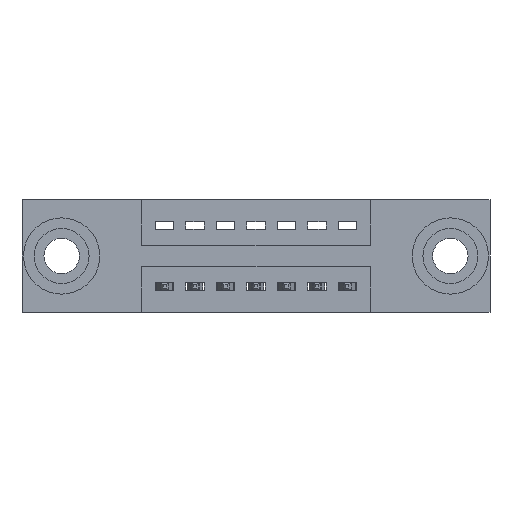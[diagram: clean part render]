
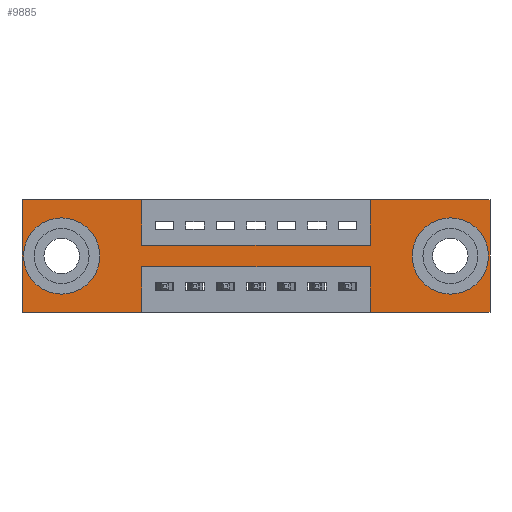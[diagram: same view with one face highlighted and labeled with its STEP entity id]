
A CAD part, front view. The second image highlights one B-rep face of the part: STEP entity #9885.
In plain terms, the highlighted planar face has unit normal (0, -1, 0).
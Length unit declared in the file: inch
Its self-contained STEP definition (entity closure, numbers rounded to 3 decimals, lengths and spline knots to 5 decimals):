
#82 = VERTEX_POINT ( 'NONE', #1654 ) ;
#415 = EDGE_CURVE ( 'NONE', #9062, #1113, #5996, .T. ) ;
#456 = ORIENTED_EDGE ( 'NONE', *, *, #10142, .F. ) ;
#490 = CARTESIAN_POINT ( 'NONE',  ( 0.13, 0., -0.263 ) ) ;
#629 = VERTEX_POINT ( 'NONE', #3877 ) ;
#755 = DIRECTION ( 'NONE',  ( 0., 0., -1. ) ) ;
#882 = VECTOR ( 'NONE', #6548, 39.37008 ) ;
#938 = CARTESIAN_POINT ( 'NONE',  ( 0.3925, 0., -0.15 ) ) ;
#989 = VERTEX_POINT ( 'NONE', #1128 ) ;
#1016 = DIRECTION ( 'NONE',  ( 0., 0., -1. ) ) ;
#1083 = ORIENTED_EDGE ( 'NONE', *, *, #5784, .F. ) ;
#1094 = CARTESIAN_POINT ( 'NONE',  ( 1.1425, 0., -0.22 ) ) ;
#1100 = AXIS2_PLACEMENT_3D ( 'NONE', #1557, #7455, #2564 ) ;
#1113 = VERTEX_POINT ( 'NONE', #490 ) ;
#1128 = CARTESIAN_POINT ( 'NONE',  ( 1.405, 0., -0.107 ) ) ;
#1370 = CARTESIAN_POINT ( 'NONE',  ( 1.1425, 0., -0.37 ) ) ;
#1557 = CARTESIAN_POINT ( 'NONE',  ( 1.405, 0., -0.185 ) ) ;
#1654 = CARTESIAN_POINT ( 'NONE',  ( 0.3925, 0., -0.22 ) ) ;
#1697 = VECTOR ( 'NONE', #1016, 39.37008 ) ;
#1730 = VERTEX_POINT ( 'NONE', #938 ) ;
#1739 = EDGE_CURVE ( 'NONE', #4841, #6452, #4478, .T. ) ;
#1789 = VECTOR ( 'NONE', #4950, 39.37008 ) ;
#1843 = CIRCLE ( 'NONE', #1100, 0.078 ) ;
#2000 = VECTOR ( 'NONE', #4420, 39.37008 ) ;
#2006 = FACE_BOUND ( 'NONE', #2363, .T. ) ;
#2059 = EDGE_LOOP ( 'NONE', ( #9842, #8125, #456, #5400, #7371, #9270, #5641, #1083, #9943, #5024, #2950, #7493 ) ) ;
#2079 = DIRECTION ( 'NONE',  ( 0., 1., 0. ) ) ;
#2245 = CARTESIAN_POINT ( 'NONE',  ( 0., 0., 0. ) ) ;
#2363 = EDGE_LOOP ( 'NONE', ( #2468, #4809 ) ) ;
#2468 = ORIENTED_EDGE ( 'NONE', *, *, #7388, .T. ) ;
#2542 = CARTESIAN_POINT ( 'NONE',  ( 0., 0., -0.37 ) ) ;
#2557 = VERTEX_POINT ( 'NONE', #5149 ) ;
#2564 = DIRECTION ( 'NONE',  ( 0., 0., -1. ) ) ;
#2681 = EDGE_CURVE ( 'NONE', #82, #2557, #8882, .T. ) ;
#2788 = CARTESIAN_POINT ( 'NONE',  ( 1.1425, 0., 0. ) ) ;
#2950 = ORIENTED_EDGE ( 'NONE', *, *, #9751, .F. ) ;
#2962 = DIRECTION ( 'NONE',  ( 0., 1., 0. ) ) ;
#3237 = EDGE_CURVE ( 'NONE', #2557, #629, #6519, .T. ) ;
#3473 = AXIS2_PLACEMENT_3D ( 'NONE', #7750, #2962, #8460 ) ;
#3496 = AXIS2_PLACEMENT_3D ( 'NONE', #6977, #9857, #5509 ) ;
#3508 = CARTESIAN_POINT ( 'NONE',  ( 1.535, 0., 0. ) ) ;
#3595 = CARTESIAN_POINT ( 'NONE',  ( 0., 0., 0. ) ) ;
#3743 = DIRECTION ( 'NONE',  ( 0., 0., 1. ) ) ;
#3753 = CARTESIAN_POINT ( 'NONE',  ( 1.535, 0., 0. ) ) ;
#3757 = DIRECTION ( 'NONE',  ( 0., 1., 0. ) ) ;
#3770 = CARTESIAN_POINT ( 'NONE',  ( 0.13, 0., -0.185 ) ) ;
#3877 = CARTESIAN_POINT ( 'NONE',  ( 0., 0., -0.37 ) ) ;
#3926 = AXIS2_PLACEMENT_3D ( 'NONE', #3770, #3757, #3743 ) ;
#4138 = VERTEX_POINT ( 'NONE', #1094 ) ;
#4142 = CARTESIAN_POINT ( 'NONE',  ( 0.3925, 0., -0.22 ) ) ;
#4152 = CARTESIAN_POINT ( 'NONE',  ( 0.3925, 0., -0.37 ) ) ;
#4199 = FACE_BOUND ( 'NONE', #8728, .T. ) ;
#4329 = EDGE_CURVE ( 'NONE', #6452, #5755, #8646, .T. ) ;
#4360 = CARTESIAN_POINT ( 'NONE',  ( 1.1425, 0., 0. ) ) ;
#4420 = DIRECTION ( 'NONE',  ( -1., 0., 0. ) ) ;
#4478 = LINE ( 'NONE', #3508, #1697 ) ;
#4557 = LINE ( 'NONE', #5351, #1789 ) ;
#4621 = VECTOR ( 'NONE', #9121, 39.37008 ) ;
#4710 = PLANE ( 'NONE',  #3496 ) ;
#4809 = ORIENTED_EDGE ( 'NONE', *, *, #9693, .T. ) ;
#4841 = VERTEX_POINT ( 'NONE', #3753 ) ;
#4912 = VECTOR ( 'NONE', #9776, 39.37008 ) ;
#4950 = DIRECTION ( 'NONE',  ( 1., 0., 0. ) ) ;
#4968 = DIRECTION ( 'NONE',  ( -1., 0., 0. ) ) ;
#5024 = ORIENTED_EDGE ( 'NONE', *, *, #8645, .F. ) ;
#5037 = VERTEX_POINT ( 'NONE', #10582 ) ;
#5149 = CARTESIAN_POINT ( 'NONE',  ( 0.3925, 0., -0.37 ) ) ;
#5194 = DIRECTION ( 'NONE',  ( -1., 0., 0. ) ) ;
#5217 = ORIENTED_EDGE ( 'NONE', *, *, #8427, .T. ) ;
#5263 = LINE ( 'NONE', #3595, #6782 ) ;
#5277 = CARTESIAN_POINT ( 'NONE',  ( 0., 0., 0. ) ) ;
#5351 = CARTESIAN_POINT ( 'NONE',  ( 0.3925, 0., -0.15 ) ) ;
#5400 = ORIENTED_EDGE ( 'NONE', *, *, #4329, .F. ) ;
#5401 = EDGE_CURVE ( 'NONE', #10257, #4841, #9762, .T. ) ;
#5408 = VERTEX_POINT ( 'NONE', #9918 ) ;
#5509 = DIRECTION ( 'NONE',  ( 0., 0., -1. ) ) ;
#5545 = CARTESIAN_POINT ( 'NONE',  ( 1.1425, 0., -0.37 ) ) ;
#5547 = ORIENTED_EDGE ( 'NONE', *, *, #415, .T. ) ;
#5641 = ORIENTED_EDGE ( 'NONE', *, *, #7259, .F. ) ;
#5755 = VERTEX_POINT ( 'NONE', #5545 ) ;
#5784 = EDGE_CURVE ( 'NONE', #1730, #6793, #4557, .T. ) ;
#5996 = CIRCLE ( 'NONE', #3926, 0.078 ) ;
#6452 = VERTEX_POINT ( 'NONE', #10271 ) ;
#6519 = LINE ( 'NONE', #2542, #2000 ) ;
#6548 = DIRECTION ( 'NONE',  ( 0., 0., 1. ) ) ;
#6607 = VECTOR ( 'NONE', #4968, 39.37008 ) ;
#6782 = VECTOR ( 'NONE', #8199, 39.37008 ) ;
#6793 = VERTEX_POINT ( 'NONE', #7779 ) ;
#6933 = LINE ( 'NONE', #2788, #4912 ) ;
#6977 = CARTESIAN_POINT ( 'NONE',  ( 0., 0., -0.37 ) ) ;
#7086 = CARTESIAN_POINT ( 'NONE',  ( 1.405, 0., -0.185 ) ) ;
#7130 = AXIS2_PLACEMENT_3D ( 'NONE', #7086, #2079, #7795 ) ;
#7238 = CARTESIAN_POINT ( 'NONE',  ( 0.13, 0., -0.107 ) ) ;
#7259 = EDGE_CURVE ( 'NONE', #6793, #10257, #6933, .T. ) ;
#7358 = CIRCLE ( 'NONE', #3473, 0.078 ) ;
#7371 = ORIENTED_EDGE ( 'NONE', *, *, #1739, .F. ) ;
#7388 = EDGE_CURVE ( 'NONE', #989, #5408, #7720, .T. ) ;
#7455 = DIRECTION ( 'NONE',  ( 0., 1., 0. ) ) ;
#7493 = ORIENTED_EDGE ( 'NONE', *, *, #3237, .F. ) ;
#7720 = CIRCLE ( 'NONE', #7130, 0.078 ) ;
#7750 = CARTESIAN_POINT ( 'NONE',  ( 0.13, 0., -0.185 ) ) ;
#7779 = CARTESIAN_POINT ( 'NONE',  ( 1.1425, 0., -0.15 ) ) ;
#7795 = DIRECTION ( 'NONE',  ( 0., 0., -1. ) ) ;
#7845 = VECTOR ( 'NONE', #10093, 39.37008 ) ;
#7870 = LINE ( 'NONE', #5277, #9352 ) ;
#8125 = ORIENTED_EDGE ( 'NONE', *, *, #10658, .F. ) ;
#8181 = VECTOR ( 'NONE', #5194, 39.37008 ) ;
#8199 = DIRECTION ( 'NONE',  ( 1., 0., 0. ) ) ;
#8203 = FACE_OUTER_BOUND ( 'NONE', #2059, .T. ) ;
#8337 = LINE ( 'NONE', #8424, #4621 ) ;
#8424 = CARTESIAN_POINT ( 'NONE',  ( 0.3925, 0., 0. ) ) ;
#8427 = EDGE_CURVE ( 'NONE', #1113, #9062, #7358, .T. ) ;
#8460 = DIRECTION ( 'NONE',  ( 0., 0., 1. ) ) ;
#8522 = LINE ( 'NONE', #4142, #6607 ) ;
#8645 = EDGE_CURVE ( 'NONE', #10647, #5037, #5263, .T. ) ;
#8646 = LINE ( 'NONE', #8901, #8181 ) ;
#8672 = VECTOR ( 'NONE', #755, 39.37008 ) ;
#8728 = EDGE_LOOP ( 'NONE', ( #5547, #5217 ) ) ;
#8872 = EDGE_CURVE ( 'NONE', #5037, #1730, #8337, .T. ) ;
#8882 = LINE ( 'NONE', #4152, #8672 ) ;
#8901 = CARTESIAN_POINT ( 'NONE',  ( 0., 0., -0.37 ) ) ;
#8933 = DIRECTION ( 'NONE',  ( 0., 0., 1. ) ) ;
#9062 = VERTEX_POINT ( 'NONE', #7238 ) ;
#9121 = DIRECTION ( 'NONE',  ( 0., 0., -1. ) ) ;
#9270 = ORIENTED_EDGE ( 'NONE', *, *, #5401, .F. ) ;
#9352 = VECTOR ( 'NONE', #8933, 39.37008 ) ;
#9561 = LINE ( 'NONE', #1370, #882 ) ;
#9693 = EDGE_CURVE ( 'NONE', #5408, #989, #1843, .T. ) ;
#9751 = EDGE_CURVE ( 'NONE', #629, #10647, #7870, .T. ) ;
#9762 = LINE ( 'NONE', #9975, #7845 ) ;
#9776 = DIRECTION ( 'NONE',  ( 0., 0., 1. ) ) ;
#9842 = ORIENTED_EDGE ( 'NONE', *, *, #2681, .F. ) ;
#9857 = DIRECTION ( 'NONE',  ( 0., -1., 0. ) ) ;
#9885 = ADVANCED_FACE ( 'NONE', ( #2006, #4199, #8203 ), #4710, .T. ) ;
#9918 = CARTESIAN_POINT ( 'NONE',  ( 1.405, 0., -0.263 ) ) ;
#9943 = ORIENTED_EDGE ( 'NONE', *, *, #8872, .F. ) ;
#9975 = CARTESIAN_POINT ( 'NONE',  ( 0., 0., 0. ) ) ;
#10093 = DIRECTION ( 'NONE',  ( 1., 0., 0. ) ) ;
#10142 = EDGE_CURVE ( 'NONE', #5755, #4138, #9561, .T. ) ;
#10257 = VERTEX_POINT ( 'NONE', #4360 ) ;
#10271 = CARTESIAN_POINT ( 'NONE',  ( 1.535, 0., -0.37 ) ) ;
#10582 = CARTESIAN_POINT ( 'NONE',  ( 0.3925, 0., 0. ) ) ;
#10647 = VERTEX_POINT ( 'NONE', #2245 ) ;
#10658 = EDGE_CURVE ( 'NONE', #4138, #82, #8522, .T. ) ;
